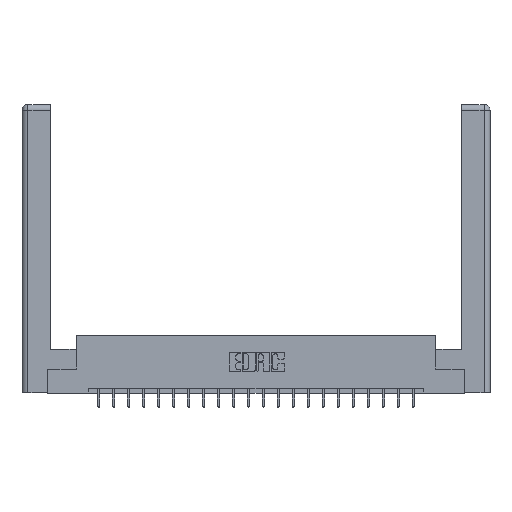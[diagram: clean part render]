
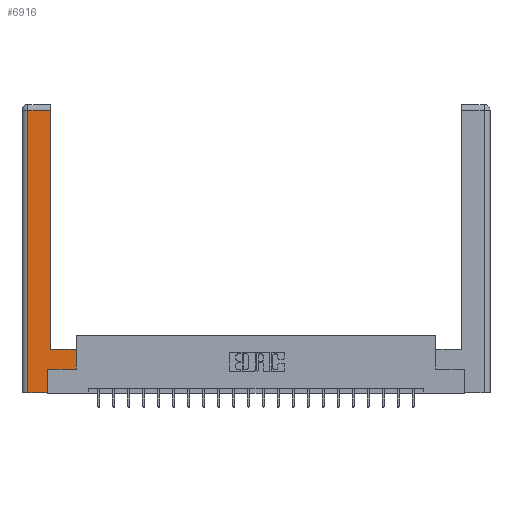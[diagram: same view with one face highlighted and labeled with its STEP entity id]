
A CAD part, top view. The second image highlights one B-rep face of the part: STEP entity #6916.
In plain terms, the highlighted planar face has unit normal (0, 0, 1).
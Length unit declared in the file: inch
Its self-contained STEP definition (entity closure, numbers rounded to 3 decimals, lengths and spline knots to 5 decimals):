
#147 = DIRECTION ( 'NONE',  ( 0., 1., 0. ) ) ;
#190 = PLANE ( 'NONE',  #9769 ) ;
#590 = VERTEX_POINT ( 'NONE', #3447 ) ;
#605 = EDGE_CURVE ( 'NONE', #15945, #11241, #14149, .T. ) ;
#656 = DIRECTION ( 'NONE',  ( 1., 0., 0. ) ) ;
#1465 = VERTEX_POINT ( 'NONE', #3563 ) ;
#1658 = EDGE_CURVE ( 'NONE', #13520, #1465, #7376, .T. ) ;
#1749 = CARTESIAN_POINT ( 'NONE',  ( 0.295, 2.94, 0. ) ) ;
#1929 = CARTESIAN_POINT ( 'NONE',  ( 0., 0., 0. ) ) ;
#2408 = LINE ( 'NONE', #21723, #10993 ) ;
#2821 = DIRECTION ( 'NONE',  ( 1., 0., 0. ) ) ;
#3014 = CARTESIAN_POINT ( 'NONE',  ( 0.0615, 0., 0. ) ) ;
#3192 = EDGE_CURVE ( 'NONE', #11813, #15945, #13196, .T. ) ;
#3447 = CARTESIAN_POINT ( 'NONE',  ( 0.565, 0.245, 0. ) ) ;
#3536 = VECTOR ( 'NONE', #656, 39.37008 ) ;
#3563 = CARTESIAN_POINT ( 'NONE',  ( 0.295, 0.45, 0. ) ) ;
#3787 = FACE_OUTER_BOUND ( 'NONE', #12188, .T. ) ;
#3933 = EDGE_CURVE ( 'NONE', #590, #13520, #17509, .T. ) ;
#4064 = ORIENTED_EDGE ( 'NONE', *, *, #3192, .T. ) ;
#4435 = VECTOR ( 'NONE', #11642, 39.37008 ) ;
#4465 = ORIENTED_EDGE ( 'NONE', *, *, #12281, .T. ) ;
#4958 = VERTEX_POINT ( 'NONE', #1749 ) ;
#5151 = DIRECTION ( 'NONE',  ( 0., 0., -1. ) ) ;
#5859 = CARTESIAN_POINT ( 'NONE',  ( 0.265, 0., 0. ) ) ;
#6916 = ADVANCED_FACE ( 'NONE', ( #3787 ), #190, .F. ) ;
#7226 = ORIENTED_EDGE ( 'NONE', *, *, #605, .T. ) ;
#7376 = LINE ( 'NONE', #9700, #13546 ) ;
#8096 = DIRECTION ( 'NONE',  ( 0., 1., 0. ) ) ;
#8137 = LINE ( 'NONE', #15658, #15396 ) ;
#8346 = VECTOR ( 'NONE', #13733, 39.37008 ) ;
#8571 = CARTESIAN_POINT ( 'NONE',  ( 0.265, 0.245, 0. ) ) ;
#9009 = ORIENTED_EDGE ( 'NONE', *, *, #3933, .T. ) ;
#9498 = CARTESIAN_POINT ( 'NONE',  ( 0.0615, 0., 0. ) ) ;
#9700 = CARTESIAN_POINT ( 'NONE',  ( 0.295, 0.45, 0. ) ) ;
#9741 = CARTESIAN_POINT ( 'NONE',  ( 0.265, 0.245, 0. ) ) ;
#9769 = AXIS2_PLACEMENT_3D ( 'NONE', #1929, #5151, #13787 ) ;
#9877 = EDGE_CURVE ( 'NONE', #13082, #11813, #20587, .T. ) ;
#10993 = VECTOR ( 'NONE', #2821, 39.37008 ) ;
#11241 = VERTEX_POINT ( 'NONE', #9741 ) ;
#11374 = VECTOR ( 'NONE', #8096, 39.37008 ) ;
#11581 = EDGE_CURVE ( 'NONE', #4958, #13082, #8137, .T. ) ;
#11642 = DIRECTION ( 'NONE',  ( 0., -1., 0. ) ) ;
#11813 = VERTEX_POINT ( 'NONE', #9498 ) ;
#12188 = EDGE_LOOP ( 'NONE', ( #4465, #20703, #13914, #4064, #7226, #19317, #9009, #18918 ) ) ;
#12281 = EDGE_CURVE ( 'NONE', #1465, #4958, #18287, .T. ) ;
#13005 = CARTESIAN_POINT ( 'NONE',  ( 0.0615, 2.94, 0. ) ) ;
#13082 = VERTEX_POINT ( 'NONE', #13005 ) ;
#13196 = LINE ( 'NONE', #5859, #3536 ) ;
#13520 = VERTEX_POINT ( 'NONE', #19888 ) ;
#13546 = VECTOR ( 'NONE', #14883, 39.37008 ) ;
#13733 = DIRECTION ( 'NONE',  ( 0., 1., 0. ) ) ;
#13787 = DIRECTION ( 'NONE',  ( -1., 0., 0. ) ) ;
#13914 = ORIENTED_EDGE ( 'NONE', *, *, #9877, .T. ) ;
#14149 = LINE ( 'NONE', #8571, #15494 ) ;
#14883 = DIRECTION ( 'NONE',  ( -1., 0., 0. ) ) ;
#15396 = VECTOR ( 'NONE', #15737, 39.37008 ) ;
#15464 = EDGE_CURVE ( 'NONE', #11241, #590, #2408, .T. ) ;
#15494 = VECTOR ( 'NONE', #147, 39.37008 ) ;
#15658 = CARTESIAN_POINT ( 'NONE',  ( 0.0615, 2.94, 0. ) ) ;
#15737 = DIRECTION ( 'NONE',  ( -1., 0., 0. ) ) ;
#15744 = CARTESIAN_POINT ( 'NONE',  ( 0.265, 0., 0. ) ) ;
#15945 = VERTEX_POINT ( 'NONE', #15744 ) ;
#17202 = CARTESIAN_POINT ( 'NONE',  ( 0.565, 0.45, 0. ) ) ;
#17509 = LINE ( 'NONE', #17202, #8346 ) ;
#18287 = LINE ( 'NONE', #19939, #11374 ) ;
#18918 = ORIENTED_EDGE ( 'NONE', *, *, #1658, .T. ) ;
#19317 = ORIENTED_EDGE ( 'NONE', *, *, #15464, .T. ) ;
#19888 = CARTESIAN_POINT ( 'NONE',  ( 0.565, 0.45, 0. ) ) ;
#19939 = CARTESIAN_POINT ( 'NONE',  ( 0.295, 3., 0. ) ) ;
#20587 = LINE ( 'NONE', #3014, #4435 ) ;
#20703 = ORIENTED_EDGE ( 'NONE', *, *, #11581, .T. ) ;
#21723 = CARTESIAN_POINT ( 'NONE',  ( 0.565, 0.245, 0. ) ) ;
